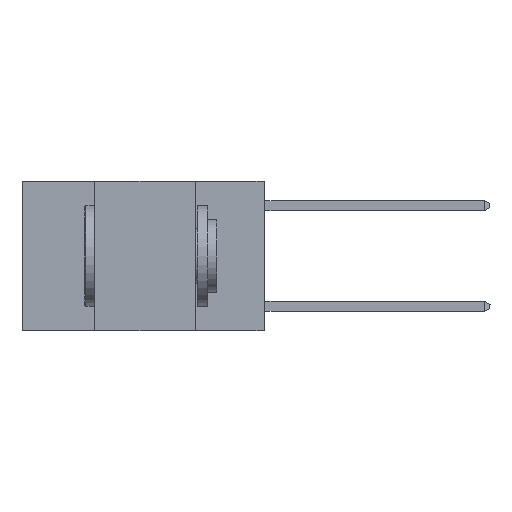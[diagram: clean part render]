
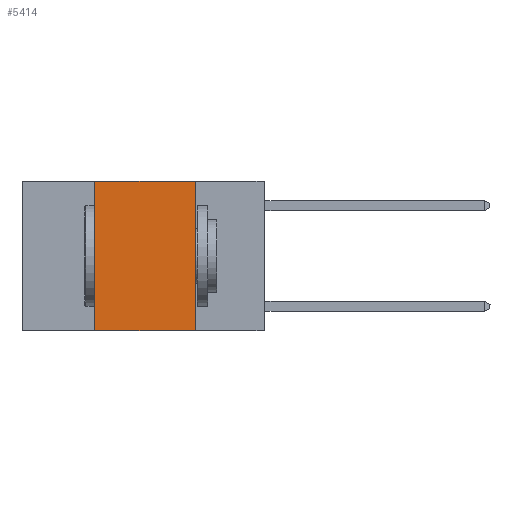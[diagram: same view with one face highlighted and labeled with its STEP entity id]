
A CAD part, left-side view. The second image highlights one B-rep face of the part: STEP entity #5414.
In plain terms, the highlighted planar face has unit normal (-1, 0, 0).
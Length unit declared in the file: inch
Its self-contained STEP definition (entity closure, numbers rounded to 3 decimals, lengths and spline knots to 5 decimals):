
#107 = EDGE_CURVE ( 'NONE', #7733, #16593, #7587, .T. ) ;
#766 = LINE ( 'NONE', #15704, #8252 ) ;
#877 = VERTEX_POINT ( 'NONE', #21903 ) ;
#996 = FACE_OUTER_BOUND ( 'NONE', #19328, .T. ) ;
#2511 = VERTEX_POINT ( 'NONE', #8720 ) ;
#4036 = PLANE ( 'NONE',  #13266 ) ;
#4080 = DIRECTION ( 'NONE',  ( 0., 0., 1. ) ) ;
#5414 = ADVANCED_FACE ( 'NONE', ( #996 ), #4036, .F. ) ;
#5486 = DIRECTION ( 'NONE',  ( 0., 0., -1. ) ) ;
#6754 = DIRECTION ( 'NONE',  ( 0., -1., 0. ) ) ;
#7587 = LINE ( 'NONE', #13504, #11881 ) ;
#7733 = VERTEX_POINT ( 'NONE', #8174 ) ;
#8138 = EDGE_CURVE ( 'NONE', #7733, #2511, #9975, .T. ) ;
#8174 = CARTESIAN_POINT ( 'NONE',  ( 0., 0.42, -0.37 ) ) ;
#8252 = VECTOR ( 'NONE', #5486, 39.37008 ) ;
#8325 = VECTOR ( 'NONE', #6754, 39.37008 ) ;
#8720 = CARTESIAN_POINT ( 'NONE',  ( 0., 0.42, 0. ) ) ;
#9156 = DIRECTION ( 'NONE',  ( 1., 0., 0. ) ) ;
#9975 = LINE ( 'NONE', #12573, #10495 ) ;
#10259 = EDGE_CURVE ( 'NONE', #2511, #877, #13418, .T. ) ;
#10495 = VECTOR ( 'NONE', #4080, 39.37008 ) ;
#11881 = VECTOR ( 'NONE', #21897, 39.37008 ) ;
#12573 = CARTESIAN_POINT ( 'NONE',  ( 0., 0.42, 0. ) ) ;
#12915 = CARTESIAN_POINT ( 'NONE',  ( 0., 0.17, -0.37 ) ) ;
#13266 = AXIS2_PLACEMENT_3D ( 'NONE', #15973, #9156, #21016 ) ;
#13418 = LINE ( 'NONE', #16969, #8325 ) ;
#13504 = CARTESIAN_POINT ( 'NONE',  ( 0., 0.6, -0.37 ) ) ;
#15704 = CARTESIAN_POINT ( 'NONE',  ( 0., 0.17, 0. ) ) ;
#15973 = CARTESIAN_POINT ( 'NONE',  ( 0., 0.6, 0. ) ) ;
#16593 = VERTEX_POINT ( 'NONE', #12915 ) ;
#16969 = CARTESIAN_POINT ( 'NONE',  ( 0., 0.6, 0. ) ) ;
#18005 = ORIENTED_EDGE ( 'NONE', *, *, #21055, .F. ) ;
#19328 = EDGE_LOOP ( 'NONE', ( #18005, #20115, #21644, #20369 ) ) ;
#20115 = ORIENTED_EDGE ( 'NONE', *, *, #10259, .F. ) ;
#20369 = ORIENTED_EDGE ( 'NONE', *, *, #107, .T. ) ;
#21016 = DIRECTION ( 'NONE',  ( 0., 0., -1. ) ) ;
#21055 = EDGE_CURVE ( 'NONE', #877, #16593, #766, .T. ) ;
#21644 = ORIENTED_EDGE ( 'NONE', *, *, #8138, .F. ) ;
#21897 = DIRECTION ( 'NONE',  ( 0., -1., 0. ) ) ;
#21903 = CARTESIAN_POINT ( 'NONE',  ( 0., 0.17, 0. ) ) ;
